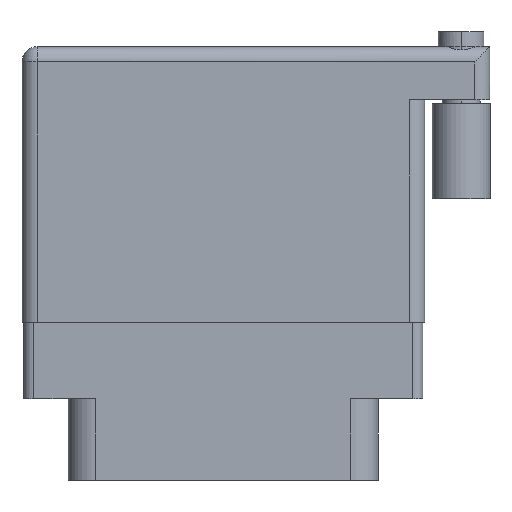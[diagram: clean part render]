
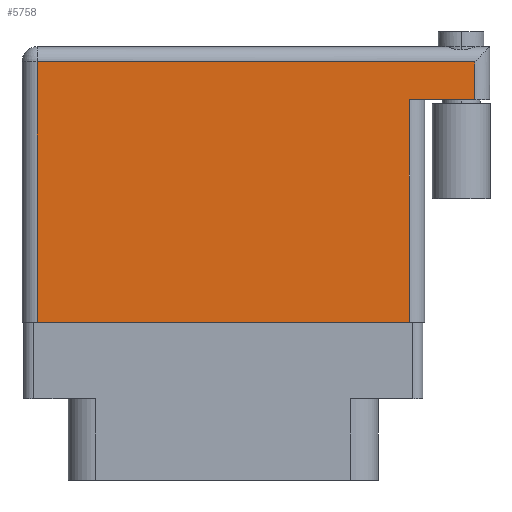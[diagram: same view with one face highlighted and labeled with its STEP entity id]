
A CAD part, front view. The second image highlights one B-rep face of the part: STEP entity #5758.
In plain terms, the highlighted face is planar.
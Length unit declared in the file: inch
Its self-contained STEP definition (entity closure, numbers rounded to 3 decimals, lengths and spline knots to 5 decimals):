
#24 = DIRECTION ( 'NONE',  ( 0., 0., -1. ) ) ;
#432 = VECTOR ( 'NONE', #3510, 39.37008 ) ;
#450 = CARTESIAN_POINT ( 'NONE',  ( 0., 0., 0. ) ) ;
#2623 = VECTOR ( 'NONE', #10285, 39.37008 ) ;
#3317 = CARTESIAN_POINT ( 'NONE',  ( 1.489, 0.856, 0. ) ) ;
#3510 = DIRECTION ( 'NONE',  ( 0., -1., 0. ) ) ;
#3725 = EDGE_CURVE ( 'NONE', #11018, #7375, #5924, .T. ) ;
#3820 = EDGE_CURVE ( 'NONE', #12951, #25424, #14358, .T. ) ;
#4281 = EDGE_CURVE ( 'NONE', #14359, #12951, #5495, .T. ) ;
#4411 = EDGE_LOOP ( 'NONE', ( #24187, #24089, #10622, #11733, #14908, #14830 ) ) ;
#4664 = VECTOR ( 'NONE', #21730, 39.37008 ) ;
#4838 = CARTESIAN_POINT ( 'NONE',  ( 1.275, 0.731, 0. ) ) ;
#5495 = LINE ( 'NONE', #13676, #432 ) ;
#5758 = ADVANCED_FACE ( 'NONE', ( #21014 ), #8727, .F. ) ;
#5924 = LINE ( 'NONE', #9687, #10653 ) ;
#7375 = VERTEX_POINT ( 'NONE', #7406 ) ;
#7406 = CARTESIAN_POINT ( 'NONE',  ( 1.275, 0.731, 0. ) ) ;
#8082 = DIRECTION ( 'NONE',  ( 0., 1., 0. ) ) ;
#8131 = CARTESIAN_POINT ( 'NONE',  ( 0., 0.856, 0. ) ) ;
#8727 = PLANE ( 'NONE',  #18792 ) ;
#9317 = LINE ( 'NONE', #25607, #4664 ) ;
#9613 = CARTESIAN_POINT ( 'NONE',  ( 0.05, 0., 0. ) ) ;
#9687 = CARTESIAN_POINT ( 'NONE',  ( 1.539, 0.731, 0. ) ) ;
#9962 = DIRECTION ( 'NONE',  ( -1., 0., 0. ) ) ;
#10133 = LINE ( 'NONE', #8131, #2623 ) ;
#10285 = DIRECTION ( 'NONE',  ( -1., 0., 0. ) ) ;
#10527 = EDGE_CURVE ( 'NONE', #25424, #7375, #18224, .T. ) ;
#10622 = ORIENTED_EDGE ( 'NONE', *, *, #3725, .F. ) ;
#10653 = VECTOR ( 'NONE', #9962, 39.37008 ) ;
#11018 = VERTEX_POINT ( 'NONE', #15227 ) ;
#11335 = EDGE_CURVE ( 'NONE', #12970, #14359, #10133, .T. ) ;
#11733 = ORIENTED_EDGE ( 'NONE', *, *, #14625, .T. ) ;
#12951 = VERTEX_POINT ( 'NONE', #9613 ) ;
#12970 = VERTEX_POINT ( 'NONE', #3317 ) ;
#13676 = CARTESIAN_POINT ( 'NONE',  ( 0.05, 0., 0. ) ) ;
#14358 = LINE ( 'NONE', #450, #16639 ) ;
#14359 = VERTEX_POINT ( 'NONE', #16413 ) ;
#14625 = EDGE_CURVE ( 'NONE', #11018, #12970, #9317, .T. ) ;
#14830 = ORIENTED_EDGE ( 'NONE', *, *, #4281, .T. ) ;
#14908 = ORIENTED_EDGE ( 'NONE', *, *, #11335, .T. ) ;
#15227 = CARTESIAN_POINT ( 'NONE',  ( 1.489, 0.731, 0. ) ) ;
#16413 = CARTESIAN_POINT ( 'NONE',  ( 0.05, 0.856, 0. ) ) ;
#16628 = DIRECTION ( 'NONE',  ( 1., 0., 0. ) ) ;
#16639 = VECTOR ( 'NONE', #16628, 39.37008 ) ;
#18224 = LINE ( 'NONE', #4838, #24801 ) ;
#18792 = AXIS2_PLACEMENT_3D ( 'NONE', #24996, #24, #24481 ) ;
#21014 = FACE_OUTER_BOUND ( 'NONE', #4411, .T. ) ;
#21639 = CARTESIAN_POINT ( 'NONE',  ( 1.275, 0., 0. ) ) ;
#21730 = DIRECTION ( 'NONE',  ( 0., 1., 0. ) ) ;
#24089 = ORIENTED_EDGE ( 'NONE', *, *, #10527, .T. ) ;
#24187 = ORIENTED_EDGE ( 'NONE', *, *, #3820, .T. ) ;
#24481 = DIRECTION ( 'NONE',  ( -1., 0., 0. ) ) ;
#24801 = VECTOR ( 'NONE', #8082, 39.37008 ) ;
#24996 = CARTESIAN_POINT ( 'NONE',  ( 0., 0.906, 0. ) ) ;
#25424 = VERTEX_POINT ( 'NONE', #21639 ) ;
#25607 = CARTESIAN_POINT ( 'NONE',  ( 1.489, 0.906, 0. ) ) ;
